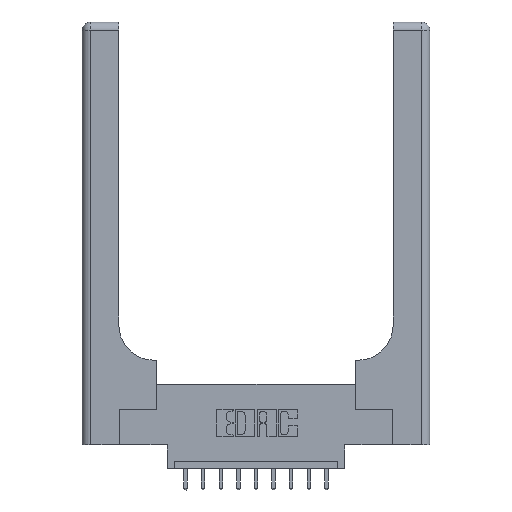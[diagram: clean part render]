
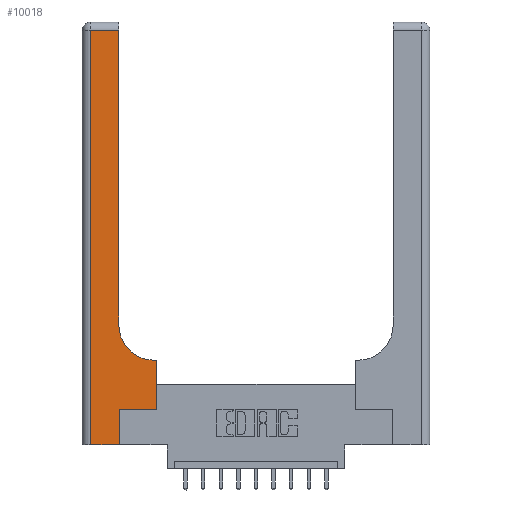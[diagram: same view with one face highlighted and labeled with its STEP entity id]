
A CAD part, top view. The second image highlights one B-rep face of the part: STEP entity #10018.
In plain terms, the highlighted planar face has unit normal (0, 0, 1).
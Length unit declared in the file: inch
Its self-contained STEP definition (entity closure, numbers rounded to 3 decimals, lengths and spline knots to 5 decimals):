
#493 = EDGE_CURVE ( 'NONE', #14268, #6150, #5702, .T. ) ;
#669 = DIRECTION ( 'NONE',  ( -1., 0., 0. ) ) ;
#806 = VERTEX_POINT ( 'NONE', #13027 ) ;
#1070 = CARTESIAN_POINT ( 'NONE',  ( 0.51, 0.6, 0.37 ) ) ;
#1220 = ORIENTED_EDGE ( 'NONE', *, *, #493, .T. ) ;
#1353 = EDGE_CURVE ( 'NONE', #806, #13561, #6789, .T. ) ;
#1477 = DIRECTION ( 'NONE',  ( 0., 0., -1. ) ) ;
#1976 = VECTOR ( 'NONE', #4763, 39.37008 ) ;
#2165 = LINE ( 'NONE', #3618, #12926 ) ;
#2844 = CARTESIAN_POINT ( 'NONE',  ( 0.26, 0.85, 0.37 ) ) ;
#2972 = CARTESIAN_POINT ( 'NONE',  ( 0.265, 0., 0.37 ) ) ;
#3618 = CARTESIAN_POINT ( 'NONE',  ( 0.06, 3., 0.37 ) ) ;
#4319 = ORIENTED_EDGE ( 'NONE', *, *, #1353, .T. ) ;
#4763 = DIRECTION ( 'NONE',  ( 0., 1., 0. ) ) ;
#5056 = DIRECTION ( 'NONE',  ( 1., 0., 0. ) ) ;
#5238 = CARTESIAN_POINT ( 'NONE',  ( 0.26, 3., 0.37 ) ) ;
#5263 = DIRECTION ( 'NONE',  ( -1., 0., 0. ) ) ;
#5324 = CARTESIAN_POINT ( 'NONE',  ( 0.06, 2.94, 0.37 ) ) ;
#5410 = EDGE_LOOP ( 'NONE', ( #7852, #7401, #7994, #8232, #1220, #13026, #4319, #9952, #13213 ) ) ;
#5702 = LINE ( 'NONE', #2972, #9220 ) ;
#5704 = CIRCLE ( 'NONE', #12236, 0.25 ) ;
#5906 = VERTEX_POINT ( 'NONE', #10898 ) ;
#6119 = DIRECTION ( 'NONE',  ( -1., 0., 0. ) ) ;
#6150 = VERTEX_POINT ( 'NONE', #12921 ) ;
#6344 = DIRECTION ( 'NONE',  ( 0., 1., 0. ) ) ;
#6524 = VERTEX_POINT ( 'NONE', #2844 ) ;
#6546 = LINE ( 'NONE', #9263, #14541 ) ;
#6690 = VECTOR ( 'NONE', #5056, 39.37008 ) ;
#6733 = EDGE_CURVE ( 'NONE', #13163, #6524, #5704, .T. ) ;
#6789 = LINE ( 'NONE', #15275, #1976 ) ;
#6865 = VECTOR ( 'NONE', #5263, 39.37008 ) ;
#7212 = PLANE ( 'NONE',  #8446 ) ;
#7401 = ORIENTED_EDGE ( 'NONE', *, *, #13696, .T. ) ;
#7852 = ORIENTED_EDGE ( 'NONE', *, *, #11402, .T. ) ;
#7994 = ORIENTED_EDGE ( 'NONE', *, *, #8796, .T. ) ;
#8232 = ORIENTED_EDGE ( 'NONE', *, *, #13589, .T. ) ;
#8446 = AXIS2_PLACEMENT_3D ( 'NONE', #9594, #1477, #6119 ) ;
#8578 = CARTESIAN_POINT ( 'NONE',  ( 0.528, 0.6, 0.37 ) ) ;
#8796 = EDGE_CURVE ( 'NONE', #11887, #5906, #2165, .T. ) ;
#9220 = VECTOR ( 'NONE', #6344, 39.37008 ) ;
#9263 = CARTESIAN_POINT ( 'NONE',  ( 0.265, 0.25, 0.37 ) ) ;
#9525 = FACE_OUTER_BOUND ( 'NONE', #5410, .T. ) ;
#9594 = CARTESIAN_POINT ( 'NONE',  ( 0., 3., 0.37 ) ) ;
#9952 = ORIENTED_EDGE ( 'NONE', *, *, #11318, .T. ) ;
#10018 = ADVANCED_FACE ( 'NONE', ( #9525 ), #7212, .F. ) ;
#10063 = DIRECTION ( 'NONE',  ( 0., 1., 0. ) ) ;
#10407 = LINE ( 'NONE', #14816, #6865 ) ;
#10474 = DIRECTION ( 'NONE',  ( 1., 0., 0. ) ) ;
#10898 = CARTESIAN_POINT ( 'NONE',  ( 0.06, 0., 0.37 ) ) ;
#10946 = CARTESIAN_POINT ( 'NONE',  ( 0.265, 0., 0.37 ) ) ;
#11041 = EDGE_CURVE ( 'NONE', #6150, #806, #6546, .T. ) ;
#11318 = EDGE_CURVE ( 'NONE', #13561, #13163, #13241, .T. ) ;
#11364 = VECTOR ( 'NONE', #669, 39.37008 ) ;
#11402 = EDGE_CURVE ( 'NONE', #6524, #11436, #11726, .T. ) ;
#11436 = VERTEX_POINT ( 'NONE', #13902 ) ;
#11726 = LINE ( 'NONE', #5238, #13788 ) ;
#11887 = VERTEX_POINT ( 'NONE', #5324 ) ;
#12174 = CARTESIAN_POINT ( 'NONE',  ( 0., 0., 0.37 ) ) ;
#12236 = AXIS2_PLACEMENT_3D ( 'NONE', #12657, #13851, #12706 ) ;
#12651 = LINE ( 'NONE', #12174, #6690 ) ;
#12657 = CARTESIAN_POINT ( 'NONE',  ( 0.51, 0.85, 0.37 ) ) ;
#12706 = DIRECTION ( 'NONE',  ( 1., 0., 0. ) ) ;
#12921 = CARTESIAN_POINT ( 'NONE',  ( 0.265, 0.25, 0.37 ) ) ;
#12926 = VECTOR ( 'NONE', #13132, 39.37008 ) ;
#13026 = ORIENTED_EDGE ( 'NONE', *, *, #11041, .T. ) ;
#13027 = CARTESIAN_POINT ( 'NONE',  ( 0.528, 0.25, 0.37 ) ) ;
#13132 = DIRECTION ( 'NONE',  ( 0., -1., 0. ) ) ;
#13163 = VERTEX_POINT ( 'NONE', #1070 ) ;
#13213 = ORIENTED_EDGE ( 'NONE', *, *, #6733, .T. ) ;
#13241 = LINE ( 'NONE', #14636, #11364 ) ;
#13561 = VERTEX_POINT ( 'NONE', #8578 ) ;
#13589 = EDGE_CURVE ( 'NONE', #5906, #14268, #12651, .T. ) ;
#13696 = EDGE_CURVE ( 'NONE', #11436, #11887, #10407, .T. ) ;
#13788 = VECTOR ( 'NONE', #10063, 39.37008 ) ;
#13851 = DIRECTION ( 'NONE',  ( 0., 0., -1. ) ) ;
#13902 = CARTESIAN_POINT ( 'NONE',  ( 0.26, 2.94, 0.37 ) ) ;
#14268 = VERTEX_POINT ( 'NONE', #10946 ) ;
#14541 = VECTOR ( 'NONE', #10474, 39.37008 ) ;
#14636 = CARTESIAN_POINT ( 'NONE',  ( 0.26, 0.6, 0.37 ) ) ;
#14816 = CARTESIAN_POINT ( 'NONE',  ( 0., 2.94, 0.37 ) ) ;
#15275 = CARTESIAN_POINT ( 'NONE',  ( 0.528, 0.25, 0.37 ) ) ;
